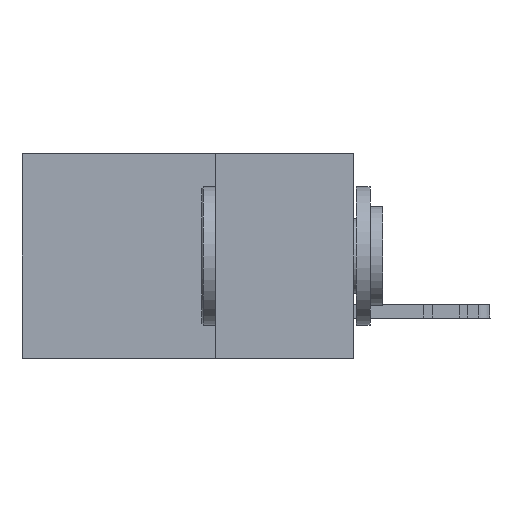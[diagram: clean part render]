
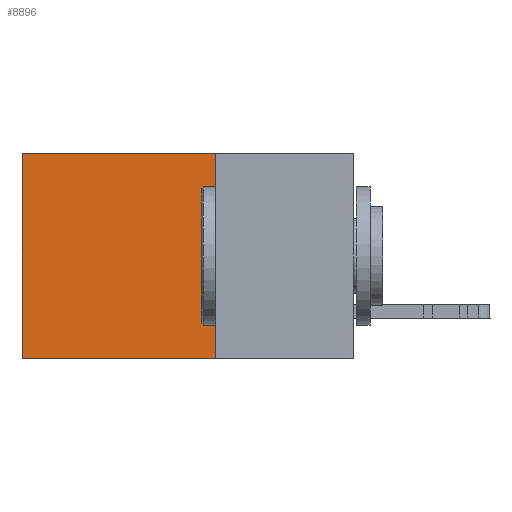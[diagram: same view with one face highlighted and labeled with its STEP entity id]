
A CAD part, left-side view. The second image highlights one B-rep face of the part: STEP entity #8896.
In plain terms, the highlighted planar face has unit normal (-1, 0, 0).
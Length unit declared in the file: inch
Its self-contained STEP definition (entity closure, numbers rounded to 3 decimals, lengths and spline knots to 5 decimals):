
#92 = EDGE_CURVE ( 'NONE', #5157, #39124, #48590, .T. ) ;
#1119 = VECTOR ( 'NONE', #34632, 39.37008 ) ;
#1506 = CARTESIAN_POINT ( 'NONE',  ( 0.2875, 0.25, 0. ) ) ;
#5157 = VERTEX_POINT ( 'NONE', #15916 ) ;
#6991 = CARTESIAN_POINT ( 'NONE',  ( 0.2875, 0.6, 0. ) ) ;
#8896 = ADVANCED_FACE ( 'NONE', ( #23747 ), #12914, .F. ) ;
#10179 = EDGE_CURVE ( 'NONE', #28308, #39124, #12250, .T. ) ;
#12250 = LINE ( 'NONE', #34794, #33594 ) ;
#12914 = PLANE ( 'NONE',  #28080 ) ;
#13647 = EDGE_CURVE ( 'NONE', #16073, #28308, #40454, .T. ) ;
#15916 = CARTESIAN_POINT ( 'NONE',  ( 0.2875, 0.6, 0. ) ) ;
#15948 = DIRECTION ( 'NONE',  ( 0., 1., 0. ) ) ;
#16073 = VERTEX_POINT ( 'NONE', #17113 ) ;
#17113 = CARTESIAN_POINT ( 'NONE',  ( 0.2875, 0.25, 0. ) ) ;
#20193 = CARTESIAN_POINT ( 'NONE',  ( 0.2875, 0.25, 0. ) ) ;
#20919 = DIRECTION ( 'NONE',  ( 1., 0., 0. ) ) ;
#23747 = FACE_OUTER_BOUND ( 'NONE', #26154, .T. ) ;
#24171 = DIRECTION ( 'NONE',  ( 0., 0., -1. ) ) ;
#26154 = EDGE_LOOP ( 'NONE', ( #29446, #30427, #46066, #36888 ) ) ;
#27243 = LINE ( 'NONE', #20193, #39937 ) ;
#28080 = AXIS2_PLACEMENT_3D ( 'NONE', #40077, #20919, #24171 ) ;
#28308 = VERTEX_POINT ( 'NONE', #29216 ) ;
#29216 = CARTESIAN_POINT ( 'NONE',  ( 0.2875, 0.25, -0.37 ) ) ;
#29446 = ORIENTED_EDGE ( 'NONE', *, *, #92, .T. ) ;
#30427 = ORIENTED_EDGE ( 'NONE', *, *, #10179, .F. ) ;
#32894 = VECTOR ( 'NONE', #50135, 39.37008 ) ;
#33594 = VECTOR ( 'NONE', #46622, 39.37008 ) ;
#34632 = DIRECTION ( 'NONE',  ( 0., 0., -1. ) ) ;
#34794 = CARTESIAN_POINT ( 'NONE',  ( 0.2875, 0.25, -0.37 ) ) ;
#36888 = ORIENTED_EDGE ( 'NONE', *, *, #45092, .T. ) ;
#39124 = VERTEX_POINT ( 'NONE', #47303 ) ;
#39937 = VECTOR ( 'NONE', #15948, 39.37008 ) ;
#40077 = CARTESIAN_POINT ( 'NONE',  ( 0.2875, 0.25, 0. ) ) ;
#40454 = LINE ( 'NONE', #1506, #1119 ) ;
#45092 = EDGE_CURVE ( 'NONE', #16073, #5157, #27243, .T. ) ;
#46066 = ORIENTED_EDGE ( 'NONE', *, *, #13647, .F. ) ;
#46622 = DIRECTION ( 'NONE',  ( 0., 1., 0. ) ) ;
#47303 = CARTESIAN_POINT ( 'NONE',  ( 0.2875, 0.6, -0.37 ) ) ;
#48590 = LINE ( 'NONE', #6991, #32894 ) ;
#50135 = DIRECTION ( 'NONE',  ( 0., 0., -1. ) ) ;
